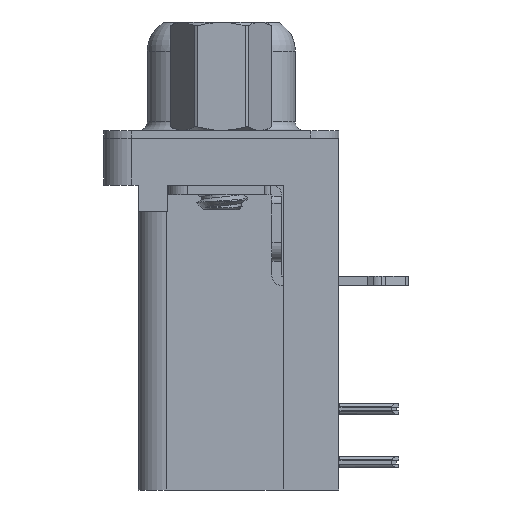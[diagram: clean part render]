
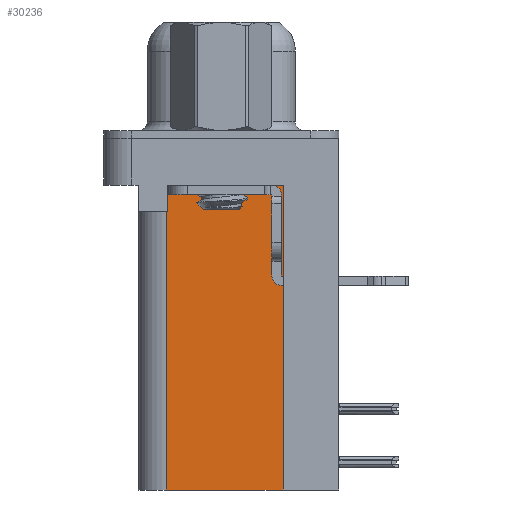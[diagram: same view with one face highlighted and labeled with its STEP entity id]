
A CAD part, left-side view. The second image highlights one B-rep face of the part: STEP entity #30236.
In plain terms, the highlighted planar face has unit normal (-1, 0, 0).
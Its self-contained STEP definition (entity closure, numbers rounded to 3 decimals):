
#527 = VERTEX_POINT ( 'NONE', #31860 ) ;
#827 = CARTESIAN_POINT ( 'NONE',  ( 3.7, -3.295, -18.76 ) ) ;
#1020 = LINE ( 'NONE', #28280, #12217 ) ;
#1579 = CARTESIAN_POINT ( 'NONE',  ( 3.7, 2.895, -3.9 ) ) ;
#2039 = VERTEX_POINT ( 'NONE', #13487 ) ;
#3086 = CARTESIAN_POINT ( 'NONE',  ( 3.7, 0., -3.9 ) ) ;
#3318 = LINE ( 'NONE', #32924, #29828 ) ;
#3843 = EDGE_CURVE ( 'NONE', #527, #8439, #27665, .T. ) ;
#4701 = VECTOR ( 'NONE', #29119, 1000. ) ;
#5096 = EDGE_CURVE ( 'NONE', #27440, #25544, #5517, .T. ) ;
#5517 = LINE ( 'NONE', #827, #4701 ) ;
#6839 = ORIENTED_EDGE ( 'NONE', *, *, #10936, .T. ) ;
#7182 = VECTOR ( 'NONE', #23494, 1000. ) ;
#7657 = EDGE_CURVE ( 'NONE', #17795, #527, #25870, .T. ) ;
#8439 = VERTEX_POINT ( 'NONE', #23693 ) ;
#8841 = CARTESIAN_POINT ( 'NONE',  ( 3.7, -3.295, -18.76 ) ) ;
#9614 = VECTOR ( 'NONE', #25312, 1000. ) ;
#10936 = EDGE_CURVE ( 'NONE', #2039, #17795, #16374, .T. ) ;
#12217 = VECTOR ( 'NONE', #30884, 1000. ) ;
#12647 = ORIENTED_EDGE ( 'NONE', *, *, #17693, .T. ) ;
#13487 = CARTESIAN_POINT ( 'NONE',  ( 3.7, -3.295, -2.5 ) ) ;
#13963 = DIRECTION ( 'NONE',  ( 0., 1., 0. ) ) ;
#14672 = EDGE_LOOP ( 'NONE', ( #6839, #18874, #29017, #23962, #22790, #12647 ) ) ;
#15488 = EDGE_CURVE ( 'NONE', #25544, #8439, #1020, .T. ) ;
#16129 = CARTESIAN_POINT ( 'NONE',  ( 3.7, 2.895, -2.5 ) ) ;
#16374 = LINE ( 'NONE', #30449, #9614 ) ;
#16851 = DIRECTION ( 'NONE',  ( 0., 0., -1. ) ) ;
#17693 = EDGE_CURVE ( 'NONE', #27440, #2039, #3318, .T. ) ;
#17795 = VERTEX_POINT ( 'NONE', #16129 ) ;
#18874 = ORIENTED_EDGE ( 'NONE', *, *, #7657, .T. ) ;
#18987 = VECTOR ( 'NONE', #16851, 1000. ) ;
#21567 = DIRECTION ( 'NONE',  ( 1., 0., 0. ) ) ;
#22669 = CARTESIAN_POINT ( 'NONE',  ( 3.7, -3.295, -18.76 ) ) ;
#22790 = ORIENTED_EDGE ( 'NONE', *, *, #5096, .F. ) ;
#23494 = DIRECTION ( 'NONE',  ( 0., 1., 0. ) ) ;
#23693 = CARTESIAN_POINT ( 'NONE',  ( 3.7, 2.925, -3.9 ) ) ;
#23962 = ORIENTED_EDGE ( 'NONE', *, *, #15488, .F. ) ;
#25177 = DIRECTION ( 'NONE',  ( 0., 0., 1. ) ) ;
#25312 = DIRECTION ( 'NONE',  ( 0., 1., 0. ) ) ;
#25520 = CARTESIAN_POINT ( 'NONE',  ( 3.7, 2.925, -18.76 ) ) ;
#25544 = VERTEX_POINT ( 'NONE', #25520 ) ;
#25870 = LINE ( 'NONE', #1579, #18987 ) ;
#27288 = AXIS2_PLACEMENT_3D ( 'NONE', #8841, #21567, #13963 ) ;
#27440 = VERTEX_POINT ( 'NONE', #22669 ) ;
#27665 = LINE ( 'NONE', #3086, #7182 ) ;
#28280 = CARTESIAN_POINT ( 'NONE',  ( 3.7, 2.925, -18.76 ) ) ;
#29017 = ORIENTED_EDGE ( 'NONE', *, *, #3843, .T. ) ;
#29119 = DIRECTION ( 'NONE',  ( 0., 1., 0. ) ) ;
#29415 = PLANE ( 'NONE',  #27288 ) ;
#29828 = VECTOR ( 'NONE', #25177, 1000. ) ;
#30236 = ADVANCED_FACE ( 'NONE', ( #32363 ), #29415, .F. ) ;
#30449 = CARTESIAN_POINT ( 'NONE',  ( 3.7, -3.295, -2.5 ) ) ;
#30884 = DIRECTION ( 'NONE',  ( 0., 0., 1. ) ) ;
#31860 = CARTESIAN_POINT ( 'NONE',  ( 3.7, 2.895, -3.9 ) ) ;
#32363 = FACE_OUTER_BOUND ( 'NONE', #14672, .T. ) ;
#32924 = CARTESIAN_POINT ( 'NONE',  ( 3.7, -3.295, -18.76 ) ) ;
